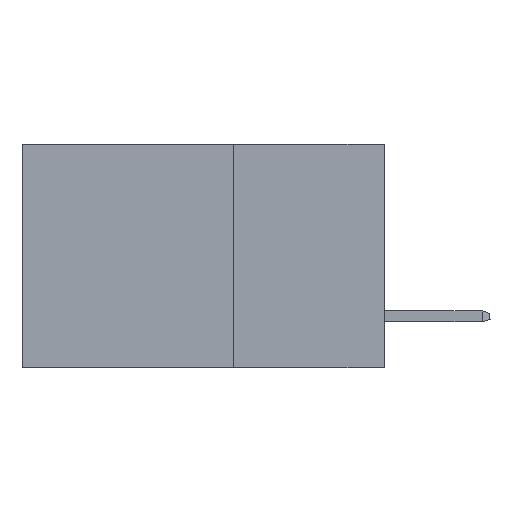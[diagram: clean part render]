
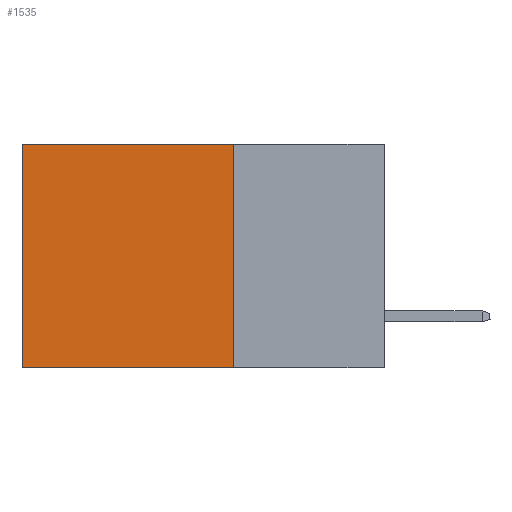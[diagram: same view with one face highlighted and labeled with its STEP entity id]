
A CAD part, left-side view. The second image highlights one B-rep face of the part: STEP entity #1535.
In plain terms, the highlighted planar face has unit normal (-1, 0, 0).
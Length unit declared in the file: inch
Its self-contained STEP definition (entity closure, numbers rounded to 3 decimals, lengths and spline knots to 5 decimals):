
#142 = ORIENTED_EDGE ( 'NONE', *, *, #161, .F. ) ;
#161 = EDGE_CURVE ( 'NONE', #11863, #6025, #731, .T. ) ;
#731 = LINE ( 'NONE', #2646, #2442 ) ;
#1535 = ADVANCED_FACE ( 'NONE', ( #19200 ), #3969, .F. ) ;
#2059 = CARTESIAN_POINT ( 'NONE',  ( 0.298, 0.6, 0. ) ) ;
#2442 = VECTOR ( 'NONE', #15220, 39.37008 ) ;
#2646 = CARTESIAN_POINT ( 'NONE',  ( 0.298, 0.25, -0.37 ) ) ;
#3969 = PLANE ( 'NONE',  #12272 ) ;
#4163 = VERTEX_POINT ( 'NONE', #13550 ) ;
#5556 = DIRECTION ( 'NONE',  ( 0., 0., -1. ) ) ;
#6025 = VERTEX_POINT ( 'NONE', #20617 ) ;
#7462 = EDGE_LOOP ( 'NONE', ( #16179, #142, #21026, #11335 ) ) ;
#8480 = LINE ( 'NONE', #15095, #11513 ) ;
#8553 = DIRECTION ( 'NONE',  ( 0., 0., -1. ) ) ;
#11136 = LINE ( 'NONE', #23214, #18747 ) ;
#11335 = ORIENTED_EDGE ( 'NONE', *, *, #18084, .T. ) ;
#11415 = EDGE_CURVE ( 'NONE', #4163, #11863, #8480, .T. ) ;
#11451 = VECTOR ( 'NONE', #15879, 39.37008 ) ;
#11513 = VECTOR ( 'NONE', #18708, 39.37008 ) ;
#11863 = VERTEX_POINT ( 'NONE', #18515 ) ;
#12027 = LINE ( 'NONE', #15720, #11451 ) ;
#12272 = AXIS2_PLACEMENT_3D ( 'NONE', #14496, #21926, #5556 ) ;
#13550 = CARTESIAN_POINT ( 'NONE',  ( 0.298, 0.25, 0. ) ) ;
#13875 = EDGE_CURVE ( 'NONE', #22463, #6025, #11136, .T. ) ;
#14496 = CARTESIAN_POINT ( 'NONE',  ( 0.298, 0.25, 0. ) ) ;
#15095 = CARTESIAN_POINT ( 'NONE',  ( 0.298, 0.25, 0. ) ) ;
#15220 = DIRECTION ( 'NONE',  ( 0., 1., 0. ) ) ;
#15720 = CARTESIAN_POINT ( 'NONE',  ( 0.298, 0.25, 0. ) ) ;
#15879 = DIRECTION ( 'NONE',  ( 0., 1., 0. ) ) ;
#16179 = ORIENTED_EDGE ( 'NONE', *, *, #13875, .T. ) ;
#18084 = EDGE_CURVE ( 'NONE', #4163, #22463, #12027, .T. ) ;
#18515 = CARTESIAN_POINT ( 'NONE',  ( 0.298, 0.25, -0.37 ) ) ;
#18708 = DIRECTION ( 'NONE',  ( 0., 0., -1. ) ) ;
#18747 = VECTOR ( 'NONE', #8553, 39.37008 ) ;
#19200 = FACE_OUTER_BOUND ( 'NONE', #7462, .T. ) ;
#20617 = CARTESIAN_POINT ( 'NONE',  ( 0.298, 0.6, -0.37 ) ) ;
#21026 = ORIENTED_EDGE ( 'NONE', *, *, #11415, .F. ) ;
#21926 = DIRECTION ( 'NONE',  ( 1., 0., 0. ) ) ;
#22463 = VERTEX_POINT ( 'NONE', #2059 ) ;
#23214 = CARTESIAN_POINT ( 'NONE',  ( 0.298, 0.6, 0. ) ) ;
